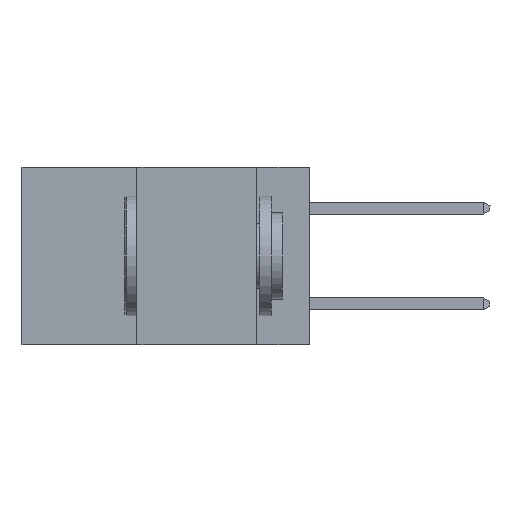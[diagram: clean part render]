
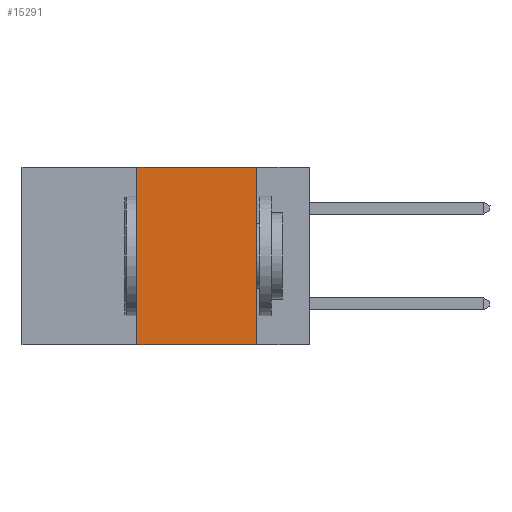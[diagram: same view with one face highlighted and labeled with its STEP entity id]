
A CAD part, left-side view. The second image highlights one B-rep face of the part: STEP entity #15291.
In plain terms, the highlighted planar face has unit normal (-1, 0, 0).
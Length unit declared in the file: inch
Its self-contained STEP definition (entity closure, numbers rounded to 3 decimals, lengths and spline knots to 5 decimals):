
#78 = DIRECTION ( 'NONE',  ( 0., -1., 0. ) ) ;
#179 = CARTESIAN_POINT ( 'NONE',  ( 0., 0.11, 0. ) ) ;
#294 = DIRECTION ( 'NONE',  ( 1., 0., 0. ) ) ;
#841 = VERTEX_POINT ( 'NONE', #2035 ) ;
#1072 = CARTESIAN_POINT ( 'NONE',  ( 0., 0.11, 0. ) ) ;
#2035 = CARTESIAN_POINT ( 'NONE',  ( 0., 0.36, -0.37 ) ) ;
#2294 = EDGE_LOOP ( 'NONE', ( #10794, #8586, #10814, #6503 ) ) ;
#2418 = FACE_OUTER_BOUND ( 'NONE', #2294, .T. ) ;
#3798 = VERTEX_POINT ( 'NONE', #179 ) ;
#4064 = CARTESIAN_POINT ( 'NONE',  ( 0., 0.36, 0. ) ) ;
#4171 = DIRECTION ( 'NONE',  ( 0., 0., 1. ) ) ;
#4936 = DIRECTION ( 'NONE',  ( 0., 0., -1. ) ) ;
#4961 = EDGE_CURVE ( 'NONE', #3798, #10809, #14471, .T. ) ;
#4981 = VERTEX_POINT ( 'NONE', #4064 ) ;
#6010 = AXIS2_PLACEMENT_3D ( 'NONE', #7705, #294, #8908 ) ;
#6284 = CARTESIAN_POINT ( 'NONE',  ( 0., 0.6, 0. ) ) ;
#6503 = ORIENTED_EDGE ( 'NONE', *, *, #15513, .T. ) ;
#7705 = CARTESIAN_POINT ( 'NONE',  ( 0., 0.6, 0. ) ) ;
#8128 = DIRECTION ( 'NONE',  ( 0., -1., 0. ) ) ;
#8253 = LINE ( 'NONE', #11302, #13415 ) ;
#8586 = ORIENTED_EDGE ( 'NONE', *, *, #11920, .F. ) ;
#8908 = DIRECTION ( 'NONE',  ( 0., 0., -1. ) ) ;
#10435 = VECTOR ( 'NONE', #78, 39.37008 ) ;
#10664 = VECTOR ( 'NONE', #4936, 39.37008 ) ;
#10794 = ORIENTED_EDGE ( 'NONE', *, *, #4961, .F. ) ;
#10809 = VERTEX_POINT ( 'NONE', #12404 ) ;
#10814 = ORIENTED_EDGE ( 'NONE', *, *, #10863, .F. ) ;
#10863 = EDGE_CURVE ( 'NONE', #841, #4981, #8253, .T. ) ;
#11156 = LINE ( 'NONE', #6284, #10435 ) ;
#11302 = CARTESIAN_POINT ( 'NONE',  ( 0., 0.36, 0. ) ) ;
#11434 = LINE ( 'NONE', #15117, #14519 ) ;
#11920 = EDGE_CURVE ( 'NONE', #4981, #3798, #11156, .T. ) ;
#12404 = CARTESIAN_POINT ( 'NONE',  ( 0., 0.11, -0.37 ) ) ;
#13415 = VECTOR ( 'NONE', #4171, 39.37008 ) ;
#13602 = PLANE ( 'NONE',  #6010 ) ;
#14471 = LINE ( 'NONE', #1072, #10664 ) ;
#14519 = VECTOR ( 'NONE', #8128, 39.37008 ) ;
#15117 = CARTESIAN_POINT ( 'NONE',  ( 0., 0.6, -0.37 ) ) ;
#15291 = ADVANCED_FACE ( 'NONE', ( #2418 ), #13602, .F. ) ;
#15513 = EDGE_CURVE ( 'NONE', #841, #10809, #11434, .T. ) ;
